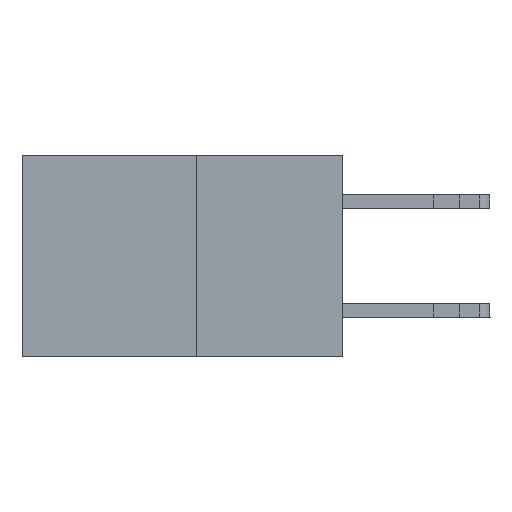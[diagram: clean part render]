
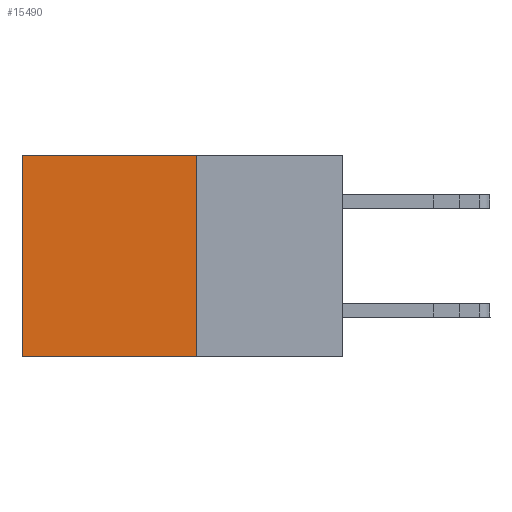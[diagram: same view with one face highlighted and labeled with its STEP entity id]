
A CAD part, left-side view. The second image highlights one B-rep face of the part: STEP entity #15490.
In plain terms, the highlighted planar face has unit normal (-1, 0, 0).
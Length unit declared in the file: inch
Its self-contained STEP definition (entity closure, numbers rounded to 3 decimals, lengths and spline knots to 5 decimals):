
#395 = VERTEX_POINT ( 'NONE', #5188 ) ;
#465 = EDGE_LOOP ( 'NONE', ( #11808, #29086, #25531, #8524 ) ) ;
#1182 = CARTESIAN_POINT ( 'NONE',  ( 0.277, 0.59, -0.37 ) ) ;
#2072 = DIRECTION ( 'NONE',  ( 1., 0., 0. ) ) ;
#3822 = DIRECTION ( 'NONE',  ( 0., 1., 0. ) ) ;
#5021 = VECTOR ( 'NONE', #3822, 39.37008 ) ;
#5188 = CARTESIAN_POINT ( 'NONE',  ( 0.277, 0.27, -0.37 ) ) ;
#6637 = CARTESIAN_POINT ( 'NONE',  ( 0.277, 0.27, -0.37 ) ) ;
#8524 = ORIENTED_EDGE ( 'NONE', *, *, #25181, .T. ) ;
#8747 = EDGE_CURVE ( 'NONE', #25620, #395, #18205, .T. ) ;
#9518 = DIRECTION ( 'NONE',  ( 0., 0., -1. ) ) ;
#10385 = VERTEX_POINT ( 'NONE', #1182 ) ;
#10507 = EDGE_CURVE ( 'NONE', #395, #10385, #29605, .T. ) ;
#10554 = LINE ( 'NONE', #12274, #22099 ) ;
#10857 = CARTESIAN_POINT ( 'NONE',  ( 0.277, 0.27, -0.37 ) ) ;
#10933 = CARTESIAN_POINT ( 'NONE',  ( 0.277, 0.27, 0. ) ) ;
#11348 = PLANE ( 'NONE',  #17128 ) ;
#11778 = VERTEX_POINT ( 'NONE', #24649 ) ;
#11808 = ORIENTED_EDGE ( 'NONE', *, *, #28985, .T. ) ;
#12107 = VECTOR ( 'NONE', #9518, 39.37008 ) ;
#12274 = CARTESIAN_POINT ( 'NONE',  ( 0.277, 0.59, -0.37 ) ) ;
#14588 = DIRECTION ( 'NONE',  ( 0., 0., -1. ) ) ;
#15490 = ADVANCED_FACE ( 'NONE', ( #18493 ), #11348, .F. ) ;
#16869 = LINE ( 'NONE', #10933, #23022 ) ;
#17128 = AXIS2_PLACEMENT_3D ( 'NONE', #6637, #2072, #18293 ) ;
#18205 = LINE ( 'NONE', #10857, #12107 ) ;
#18293 = DIRECTION ( 'NONE',  ( 0., 0., -1. ) ) ;
#18493 = FACE_OUTER_BOUND ( 'NONE', #465, .T. ) ;
#22099 = VECTOR ( 'NONE', #14588, 39.37008 ) ;
#22387 = CARTESIAN_POINT ( 'NONE',  ( 0.277, 0.27, -0.37 ) ) ;
#23022 = VECTOR ( 'NONE', #24761, 39.37008 ) ;
#24649 = CARTESIAN_POINT ( 'NONE',  ( 0.277, 0.59, 0. ) ) ;
#24761 = DIRECTION ( 'NONE',  ( 0., 1., 0. ) ) ;
#25181 = EDGE_CURVE ( 'NONE', #25620, #11778, #16869, .T. ) ;
#25531 = ORIENTED_EDGE ( 'NONE', *, *, #8747, .F. ) ;
#25620 = VERTEX_POINT ( 'NONE', #28561 ) ;
#28561 = CARTESIAN_POINT ( 'NONE',  ( 0.277, 0.27, 0. ) ) ;
#28985 = EDGE_CURVE ( 'NONE', #11778, #10385, #10554, .T. ) ;
#29086 = ORIENTED_EDGE ( 'NONE', *, *, #10507, .F. ) ;
#29605 = LINE ( 'NONE', #22387, #5021 ) ;
